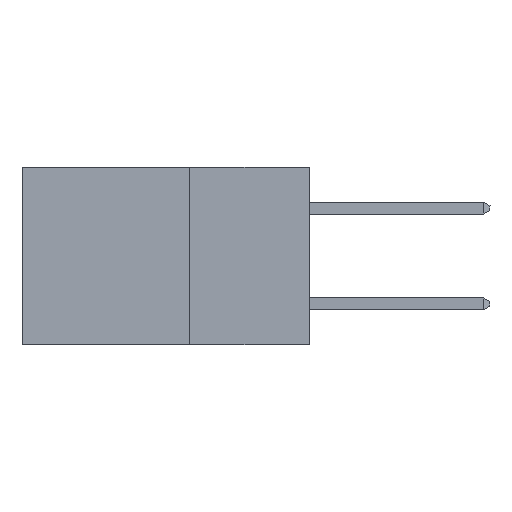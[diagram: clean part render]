
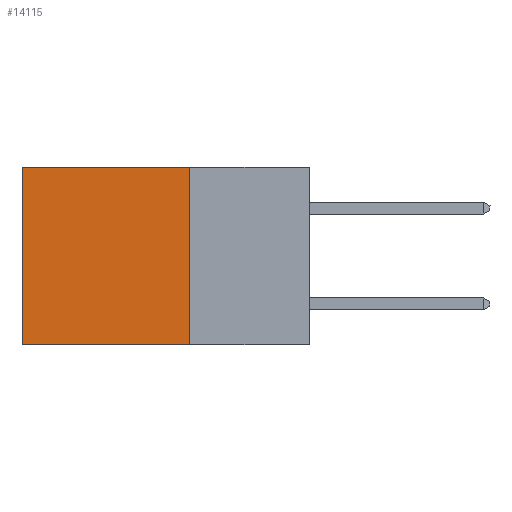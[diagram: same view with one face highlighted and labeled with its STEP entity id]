
A CAD part, left-side view. The second image highlights one B-rep face of the part: STEP entity #14115.
In plain terms, the highlighted planar face has unit normal (-1, 0, 0).
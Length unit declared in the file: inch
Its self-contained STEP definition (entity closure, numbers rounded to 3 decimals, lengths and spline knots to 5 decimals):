
#102 = DIRECTION ( 'NONE',  ( 1., 0., 0. ) ) ;
#302 = CARTESIAN_POINT ( 'NONE',  ( 0.2875, 0.6, 0. ) ) ;
#538 = FACE_OUTER_BOUND ( 'NONE', #9794, .T. ) ;
#1038 = CARTESIAN_POINT ( 'NONE',  ( 0.2875, 0.25, -0.37 ) ) ;
#1065 = EDGE_CURVE ( 'NONE', #2427, #3161, #6021, .T. ) ;
#1158 = VERTEX_POINT ( 'NONE', #1038 ) ;
#1445 = VERTEX_POINT ( 'NONE', #7716 ) ;
#1971 = DIRECTION ( 'NONE',  ( 0., 1., 0. ) ) ;
#2057 = CARTESIAN_POINT ( 'NONE',  ( 0.2875, 0.25, 0. ) ) ;
#2427 = VERTEX_POINT ( 'NONE', #7307 ) ;
#2932 = DIRECTION ( 'NONE',  ( 0., 0., -1. ) ) ;
#3161 = VERTEX_POINT ( 'NONE', #302 ) ;
#3946 = ORIENTED_EDGE ( 'NONE', *, *, #11157, .F. ) ;
#4369 = EDGE_CURVE ( 'NONE', #3161, #1445, #9155, .T. ) ;
#4761 = CARTESIAN_POINT ( 'NONE',  ( 0.2875, 0.25, 0. ) ) ;
#5177 = VECTOR ( 'NONE', #2932, 39.37008 ) ;
#5615 = VECTOR ( 'NONE', #12628, 39.37008 ) ;
#6021 = LINE ( 'NONE', #2057, #11691 ) ;
#6311 = EDGE_CURVE ( 'NONE', #2427, #1158, #8199, .T. ) ;
#7295 = ORIENTED_EDGE ( 'NONE', *, *, #1065, .T. ) ;
#7307 = CARTESIAN_POINT ( 'NONE',  ( 0.2875, 0.25, 0. ) ) ;
#7716 = CARTESIAN_POINT ( 'NONE',  ( 0.2875, 0.6, -0.37 ) ) ;
#8127 = AXIS2_PLACEMENT_3D ( 'NONE', #4761, #102, #8174 ) ;
#8174 = DIRECTION ( 'NONE',  ( 0., 0., -1. ) ) ;
#8199 = LINE ( 'NONE', #13070, #5177 ) ;
#9155 = LINE ( 'NONE', #11473, #5615 ) ;
#9422 = LINE ( 'NONE', #11569, #11696 ) ;
#9794 = EDGE_LOOP ( 'NONE', ( #12617, #3946, #12937, #7295 ) ) ;
#11157 = EDGE_CURVE ( 'NONE', #1158, #1445, #9422, .T. ) ;
#11455 = PLANE ( 'NONE',  #8127 ) ;
#11473 = CARTESIAN_POINT ( 'NONE',  ( 0.2875, 0.6, 0. ) ) ;
#11569 = CARTESIAN_POINT ( 'NONE',  ( 0.2875, 0.25, -0.37 ) ) ;
#11691 = VECTOR ( 'NONE', #1971, 39.37008 ) ;
#11696 = VECTOR ( 'NONE', #12697, 39.37008 ) ;
#12617 = ORIENTED_EDGE ( 'NONE', *, *, #4369, .T. ) ;
#12628 = DIRECTION ( 'NONE',  ( 0., 0., -1. ) ) ;
#12697 = DIRECTION ( 'NONE',  ( 0., 1., 0. ) ) ;
#12937 = ORIENTED_EDGE ( 'NONE', *, *, #6311, .F. ) ;
#13070 = CARTESIAN_POINT ( 'NONE',  ( 0.2875, 0.25, 0. ) ) ;
#14115 = ADVANCED_FACE ( 'NONE', ( #538 ), #11455, .F. ) ;
